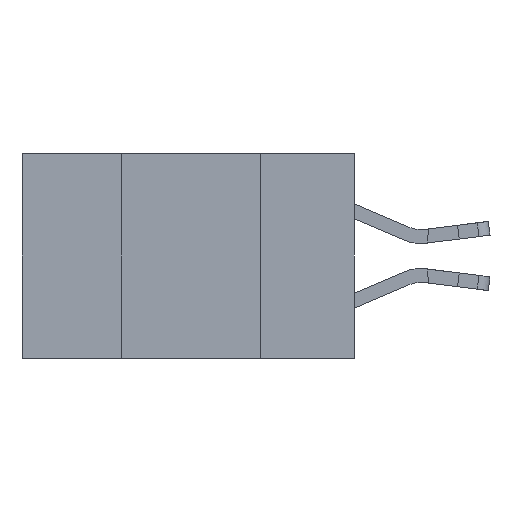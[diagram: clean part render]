
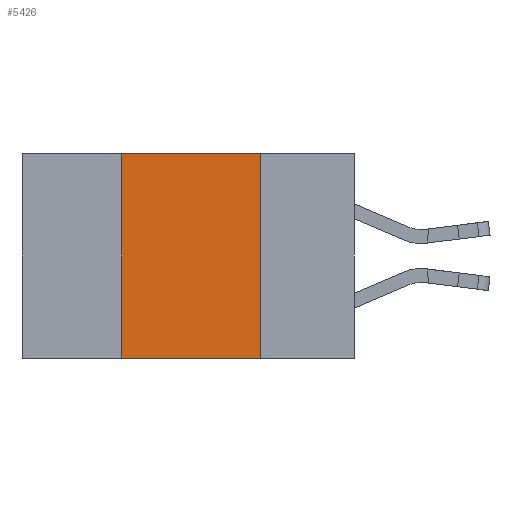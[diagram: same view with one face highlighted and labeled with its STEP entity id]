
A CAD part, left-side view. The second image highlights one B-rep face of the part: STEP entity #5426.
In plain terms, the highlighted planar face has unit normal (-1, 0, 0).
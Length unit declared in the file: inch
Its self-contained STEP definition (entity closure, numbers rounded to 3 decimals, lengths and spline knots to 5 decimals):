
#525 = LINE ( 'NONE', #1797, #1764 ) ;
#679 = CARTESIAN_POINT ( 'NONE',  ( 0., 0.17, -0.37 ) ) ;
#721 = EDGE_CURVE ( 'NONE', #15264, #10880, #2196, .T. ) ;
#908 = AXIS2_PLACEMENT_3D ( 'NONE', #16688, #9602, #9361 ) ;
#1448 = DIRECTION ( 'NONE',  ( 0., -1., 0. ) ) ;
#1764 = VECTOR ( 'NONE', #10891, 39.37008 ) ;
#1797 = CARTESIAN_POINT ( 'NONE',  ( 0., 0.6, 0. ) ) ;
#2045 = CARTESIAN_POINT ( 'NONE',  ( 0., 0.42, -0.37 ) ) ;
#2196 = LINE ( 'NONE', #16178, #5495 ) ;
#2497 = EDGE_LOOP ( 'NONE', ( #6438, #6777, #4032, #3668 ) ) ;
#3668 = ORIENTED_EDGE ( 'NONE', *, *, #10284, .T. ) ;
#4032 = ORIENTED_EDGE ( 'NONE', *, *, #6396, .F. ) ;
#4770 = VECTOR ( 'NONE', #7264, 39.37008 ) ;
#5426 = ADVANCED_FACE ( 'NONE', ( #10136 ), #6263, .F. ) ;
#5495 = VECTOR ( 'NONE', #5852, 39.37008 ) ;
#5852 = DIRECTION ( 'NONE',  ( 0., 0., -1. ) ) ;
#6263 = PLANE ( 'NONE',  #908 ) ;
#6396 = EDGE_CURVE ( 'NONE', #8833, #13344, #15139, .T. ) ;
#6438 = ORIENTED_EDGE ( 'NONE', *, *, #721, .F. ) ;
#6777 = ORIENTED_EDGE ( 'NONE', *, *, #16238, .F. ) ;
#7227 = CARTESIAN_POINT ( 'NONE',  ( 0., 0.42, 0. ) ) ;
#7264 = DIRECTION ( 'NONE',  ( 0., 0., 1. ) ) ;
#8833 = VERTEX_POINT ( 'NONE', #15035 ) ;
#9230 = VECTOR ( 'NONE', #1448, 39.37008 ) ;
#9259 = CARTESIAN_POINT ( 'NONE',  ( 0., 0.17, 0. ) ) ;
#9361 = DIRECTION ( 'NONE',  ( 0., 0., -1. ) ) ;
#9602 = DIRECTION ( 'NONE',  ( 1., 0., 0. ) ) ;
#10136 = FACE_OUTER_BOUND ( 'NONE', #2497, .T. ) ;
#10284 = EDGE_CURVE ( 'NONE', #8833, #10880, #11659, .T. ) ;
#10566 = CARTESIAN_POINT ( 'NONE',  ( 0., 0.6, -0.37 ) ) ;
#10880 = VERTEX_POINT ( 'NONE', #679 ) ;
#10891 = DIRECTION ( 'NONE',  ( 0., -1., 0. ) ) ;
#11659 = LINE ( 'NONE', #10566, #9230 ) ;
#13344 = VERTEX_POINT ( 'NONE', #7227 ) ;
#15035 = CARTESIAN_POINT ( 'NONE',  ( 0., 0.42, -0.37 ) ) ;
#15139 = LINE ( 'NONE', #2045, #4770 ) ;
#15264 = VERTEX_POINT ( 'NONE', #9259 ) ;
#16178 = CARTESIAN_POINT ( 'NONE',  ( 0., 0.17, -0.37 ) ) ;
#16238 = EDGE_CURVE ( 'NONE', #13344, #15264, #525, .T. ) ;
#16688 = CARTESIAN_POINT ( 'NONE',  ( 0., 0.6, 0. ) ) ;
